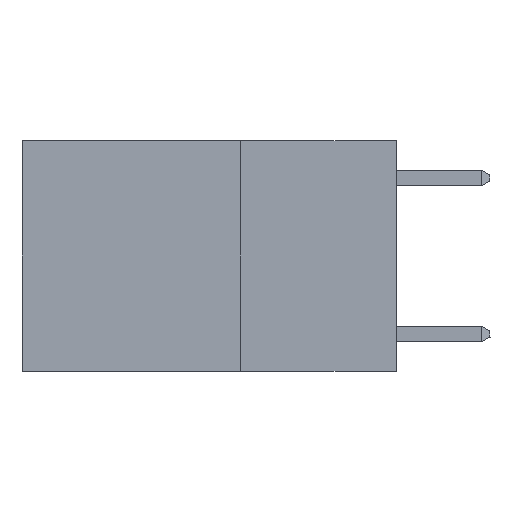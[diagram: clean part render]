
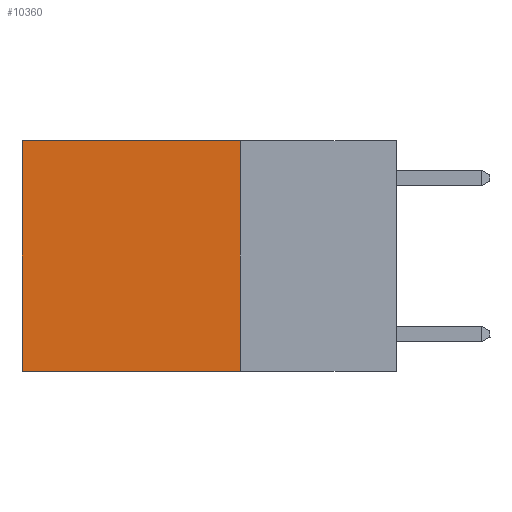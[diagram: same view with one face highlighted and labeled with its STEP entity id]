
A CAD part, left-side view. The second image highlights one B-rep face of the part: STEP entity #10360.
In plain terms, the highlighted planar face has unit normal (-1, 0, 0).
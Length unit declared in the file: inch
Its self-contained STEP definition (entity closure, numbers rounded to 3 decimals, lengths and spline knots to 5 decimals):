
#1388 = LINE ( 'NONE', #25532, #11812 ) ;
#2938 = VERTEX_POINT ( 'NONE', #24066 ) ;
#3184 = EDGE_CURVE ( 'NONE', #10721, #17415, #11147, .T. ) ;
#3636 = CARTESIAN_POINT ( 'NONE',  ( 0.2625, 0.25, 0. ) ) ;
#5180 = CARTESIAN_POINT ( 'NONE',  ( 0.2625, 0.25, 0. ) ) ;
#5366 = DIRECTION ( 'NONE',  ( 0., 0., -1. ) ) ;
#6473 = CARTESIAN_POINT ( 'NONE',  ( 0.2625, 0.6, 0. ) ) ;
#6845 = LINE ( 'NONE', #21479, #11637 ) ;
#7827 = DIRECTION ( 'NONE',  ( 0., 0., -1. ) ) ;
#9001 = CARTESIAN_POINT ( 'NONE',  ( 0.2625, 0.25, 0. ) ) ;
#9821 = ORIENTED_EDGE ( 'NONE', *, *, #3184, .T. ) ;
#10360 = ADVANCED_FACE ( 'NONE', ( #25377 ), #16024, .F. ) ;
#10721 = VERTEX_POINT ( 'NONE', #5180 ) ;
#11147 = LINE ( 'NONE', #9001, #11220 ) ;
#11220 = VECTOR ( 'NONE', #25168, 39.37008 ) ;
#11295 = DIRECTION ( 'NONE',  ( 0., 1., 0. ) ) ;
#11637 = VECTOR ( 'NONE', #11295, 39.37008 ) ;
#11812 = VECTOR ( 'NONE', #5366, 39.37008 ) ;
#13253 = ORIENTED_EDGE ( 'NONE', *, *, #17049, .F. ) ;
#14073 = EDGE_CURVE ( 'NONE', #17415, #14810, #18390, .T. ) ;
#14810 = VERTEX_POINT ( 'NONE', #18069 ) ;
#15476 = AXIS2_PLACEMENT_3D ( 'NONE', #3636, #20082, #7827 ) ;
#16024 = PLANE ( 'NONE',  #15476 ) ;
#17049 = EDGE_CURVE ( 'NONE', #10721, #2938, #1388, .T. ) ;
#17400 = ORIENTED_EDGE ( 'NONE', *, *, #25244, .F. ) ;
#17415 = VERTEX_POINT ( 'NONE', #6473 ) ;
#18069 = CARTESIAN_POINT ( 'NONE',  ( 0.2625, 0.6, -0.37 ) ) ;
#18390 = LINE ( 'NONE', #23914, #23650 ) ;
#20082 = DIRECTION ( 'NONE',  ( 1., 0., 0. ) ) ;
#21479 = CARTESIAN_POINT ( 'NONE',  ( 0.2625, 0.25, -0.37 ) ) ;
#22504 = EDGE_LOOP ( 'NONE', ( #25103, #17400, #13253, #9821 ) ) ;
#23650 = VECTOR ( 'NONE', #25830, 39.37008 ) ;
#23914 = CARTESIAN_POINT ( 'NONE',  ( 0.2625, 0.6, 0. ) ) ;
#24066 = CARTESIAN_POINT ( 'NONE',  ( 0.2625, 0.25, -0.37 ) ) ;
#25103 = ORIENTED_EDGE ( 'NONE', *, *, #14073, .T. ) ;
#25168 = DIRECTION ( 'NONE',  ( 0., 1., 0. ) ) ;
#25244 = EDGE_CURVE ( 'NONE', #2938, #14810, #6845, .T. ) ;
#25377 = FACE_OUTER_BOUND ( 'NONE', #22504, .T. ) ;
#25532 = CARTESIAN_POINT ( 'NONE',  ( 0.2625, 0.25, 0. ) ) ;
#25830 = DIRECTION ( 'NONE',  ( 0., 0., -1. ) ) ;
